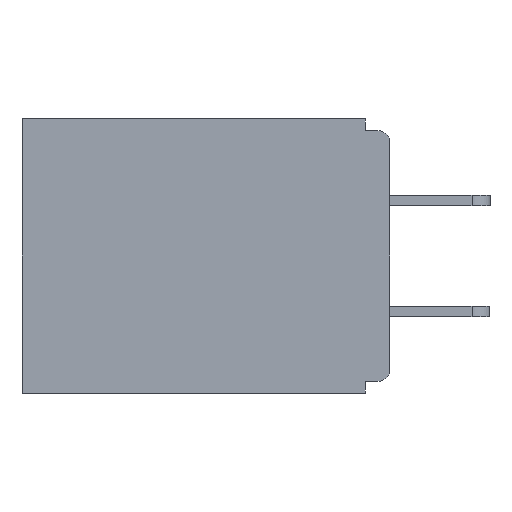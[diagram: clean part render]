
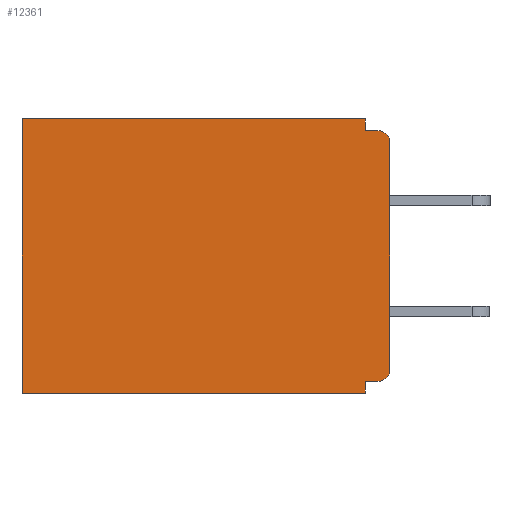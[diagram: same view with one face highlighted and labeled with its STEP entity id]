
A CAD part, left-side view. The second image highlights one B-rep face of the part: STEP entity #12361.
In plain terms, the highlighted planar face has unit normal (-1, 0, 0).
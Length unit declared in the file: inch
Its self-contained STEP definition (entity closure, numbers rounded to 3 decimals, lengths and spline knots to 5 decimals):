
#16 = VERTEX_POINT ( 'NONE', #11996 ) ;
#69 = LINE ( 'NONE', #7750, #3311 ) ;
#113 = VERTEX_POINT ( 'NONE', #9514 ) ;
#229 = PLANE ( 'NONE',  #2143 ) ;
#319 = LINE ( 'NONE', #9594, #8473 ) ;
#1148 = DIRECTION ( 'NONE',  ( 0., 0., -1. ) ) ;
#1312 = CARTESIAN_POINT ( 'NONE',  ( 0.298, 0., 0. ) ) ;
#1471 = VECTOR ( 'NONE', #3627, 39.37008 ) ;
#1863 = ORIENTED_EDGE ( 'NONE', *, *, #4800, .T. ) ;
#1900 = DIRECTION ( 'NONE',  ( 0., 1., 0. ) ) ;
#1956 = DIRECTION ( 'NONE',  ( 0., 0., -1. ) ) ;
#2139 = VECTOR ( 'NONE', #2588, 39.37008 ) ;
#2143 = AXIS2_PLACEMENT_3D ( 'NONE', #1312, #9096, #4641 ) ;
#2241 = ORIENTED_EDGE ( 'NONE', *, *, #13457, .F. ) ;
#2588 = DIRECTION ( 'NONE',  ( 0., 0., -1. ) ) ;
#2660 = FACE_OUTER_BOUND ( 'NONE', #8785, .T. ) ;
#2891 = ORIENTED_EDGE ( 'NONE', *, *, #2921, .T. ) ;
#2921 = EDGE_CURVE ( 'NONE', #16, #4206, #12873, .T. ) ;
#3073 = CARTESIAN_POINT ( 'NONE',  ( 0.298, 0.015, -0.313 ) ) ;
#3107 = DIRECTION ( 'NONE',  ( 0., 1., 0. ) ) ;
#3288 = CARTESIAN_POINT ( 'NONE',  ( 0.298, 0.031, -0.328 ) ) ;
#3311 = VECTOR ( 'NONE', #3107, 39.37008 ) ;
#3627 = DIRECTION ( 'NONE',  ( 0., -1., 0. ) ) ;
#3632 = EDGE_CURVE ( 'NONE', #113, #11656, #13849, .T. ) ;
#3817 = VECTOR ( 'NONE', #1148, 39.37008 ) ;
#3909 = VECTOR ( 'NONE', #4360, 39.37008 ) ;
#3944 = VERTEX_POINT ( 'NONE', #13181 ) ;
#4091 = CARTESIAN_POINT ( 'NONE',  ( 0.298, 0.46, -0.343 ) ) ;
#4206 = VERTEX_POINT ( 'NONE', #4091 ) ;
#4250 = LINE ( 'NONE', #8143, #1471 ) ;
#4324 = AXIS2_PLACEMENT_3D ( 'NONE', #12327, #6763, #9104 ) ;
#4360 = DIRECTION ( 'NONE',  ( 0., 1., 0. ) ) ;
#4577 = ORIENTED_EDGE ( 'NONE', *, *, #7695, .F. ) ;
#4641 = DIRECTION ( 'NONE',  ( 0., 0., -1. ) ) ;
#4729 = EDGE_CURVE ( 'NONE', #6875, #3944, #319, .T. ) ;
#4800 = EDGE_CURVE ( 'NONE', #11096, #16, #11924, .T. ) ;
#5041 = ORIENTED_EDGE ( 'NONE', *, *, #3632, .T. ) ;
#5203 = VECTOR ( 'NONE', #14175, 39.37008 ) ;
#5783 = ORIENTED_EDGE ( 'NONE', *, *, #4729, .F. ) ;
#6017 = CARTESIAN_POINT ( 'NONE',  ( 0.298, 0., 0. ) ) ;
#6024 = LINE ( 'NONE', #11982, #12090 ) ;
#6174 = AXIS2_PLACEMENT_3D ( 'NONE', #3073, #12920, #9600 ) ;
#6668 = CARTESIAN_POINT ( 'NONE',  ( 0.298, 0.46, 0. ) ) ;
#6763 = DIRECTION ( 'NONE',  ( -1., 0., 0. ) ) ;
#6875 = VERTEX_POINT ( 'NONE', #3288 ) ;
#7154 = VERTEX_POINT ( 'NONE', #8426 ) ;
#7695 = EDGE_CURVE ( 'NONE', #11096, #9012, #14230, .T. ) ;
#7750 = CARTESIAN_POINT ( 'NONE',  ( 0.298, 0., -0.343 ) ) ;
#8143 = CARTESIAN_POINT ( 'NONE',  ( 0.298, 0., -0.015 ) ) ;
#8426 = CARTESIAN_POINT ( 'NONE',  ( 0.298, 0.015, -0.328 ) ) ;
#8438 = CARTESIAN_POINT ( 'NONE',  ( 0.298, 0., 0. ) ) ;
#8473 = VECTOR ( 'NONE', #1956, 39.37008 ) ;
#8785 = EDGE_LOOP ( 'NONE', ( #5041, #9662, #4577, #1863, #2891, #2241, #5783, #11785, #10514, #11528 ) ) ;
#9012 = VERTEX_POINT ( 'NONE', #11966 ) ;
#9096 = DIRECTION ( 'NONE',  ( 1., 0., 0. ) ) ;
#9104 = DIRECTION ( 'NONE',  ( 0., 0., -1. ) ) ;
#9288 = LINE ( 'NONE', #6017, #2139 ) ;
#9514 = CARTESIAN_POINT ( 'NONE',  ( 0.298, 0., -0.03 ) ) ;
#9594 = CARTESIAN_POINT ( 'NONE',  ( 0.298, 0.031, -0.343 ) ) ;
#9600 = DIRECTION ( 'NONE',  ( 0., 0., -1. ) ) ;
#9662 = ORIENTED_EDGE ( 'NONE', *, *, #11292, .F. ) ;
#10336 = EDGE_CURVE ( 'NONE', #7154, #6875, #6024, .T. ) ;
#10514 = ORIENTED_EDGE ( 'NONE', *, *, #14029, .T. ) ;
#11096 = VERTEX_POINT ( 'NONE', #12794 ) ;
#11292 = EDGE_CURVE ( 'NONE', #9012, #11656, #4250, .T. ) ;
#11494 = CIRCLE ( 'NONE', #6174, 0.015 ) ;
#11528 = ORIENTED_EDGE ( 'NONE', *, *, #12470, .F. ) ;
#11656 = VERTEX_POINT ( 'NONE', #12318 ) ;
#11663 = VERTEX_POINT ( 'NONE', #12413 ) ;
#11785 = ORIENTED_EDGE ( 'NONE', *, *, #10336, .F. ) ;
#11924 = LINE ( 'NONE', #8438, #3909 ) ;
#11966 = CARTESIAN_POINT ( 'NONE',  ( 0.298, 0.031, -0.015 ) ) ;
#11982 = CARTESIAN_POINT ( 'NONE',  ( 0.298, 0., -0.328 ) ) ;
#11996 = CARTESIAN_POINT ( 'NONE',  ( 0.298, 0.46, 0. ) ) ;
#12090 = VECTOR ( 'NONE', #1900, 39.37008 ) ;
#12318 = CARTESIAN_POINT ( 'NONE',  ( 0.298, 0.015, -0.015 ) ) ;
#12327 = CARTESIAN_POINT ( 'NONE',  ( 0.298, 0.015, -0.03 ) ) ;
#12361 = ADVANCED_FACE ( 'NONE', ( #2660 ), #229, .F. ) ;
#12413 = CARTESIAN_POINT ( 'NONE',  ( 0.298, 0., -0.313 ) ) ;
#12470 = EDGE_CURVE ( 'NONE', #113, #11663, #9288, .T. ) ;
#12794 = CARTESIAN_POINT ( 'NONE',  ( 0.298, 0.031, 0. ) ) ;
#12873 = LINE ( 'NONE', #6668, #3817 ) ;
#12919 = CARTESIAN_POINT ( 'NONE',  ( 0.298, 0.031, -0.343 ) ) ;
#12920 = DIRECTION ( 'NONE',  ( -1., 0., 0. ) ) ;
#13181 = CARTESIAN_POINT ( 'NONE',  ( 0.298, 0.031, -0.343 ) ) ;
#13457 = EDGE_CURVE ( 'NONE', #3944, #4206, #69, .T. ) ;
#13849 = CIRCLE ( 'NONE', #4324, 0.015 ) ;
#14029 = EDGE_CURVE ( 'NONE', #7154, #11663, #11494, .T. ) ;
#14175 = DIRECTION ( 'NONE',  ( 0., 0., -1. ) ) ;
#14230 = LINE ( 'NONE', #12919, #5203 ) ;
